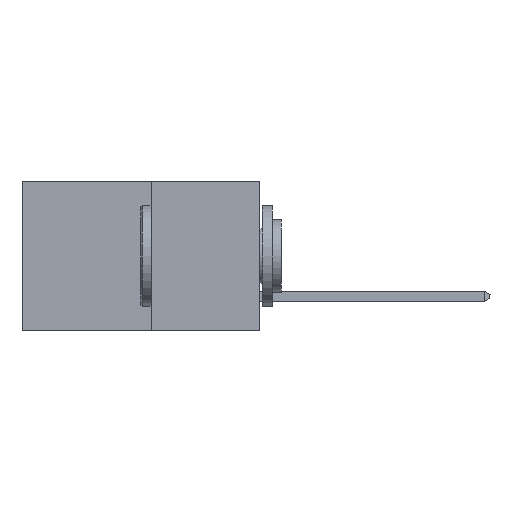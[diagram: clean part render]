
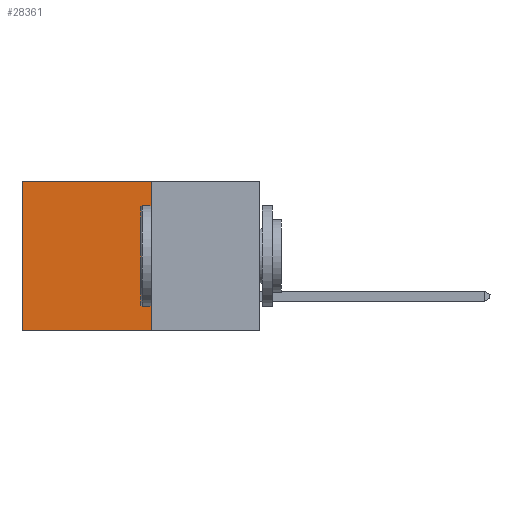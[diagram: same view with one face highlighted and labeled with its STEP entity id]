
A CAD part, left-side view. The second image highlights one B-rep face of the part: STEP entity #28361.
In plain terms, the highlighted planar face has unit normal (-1, 0, 0).
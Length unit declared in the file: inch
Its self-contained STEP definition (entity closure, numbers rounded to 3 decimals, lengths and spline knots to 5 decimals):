
#1286 = VERTEX_POINT ( 'NONE', #1595 ) ;
#1595 = CARTESIAN_POINT ( 'NONE',  ( 0.277, 0.27, 0. ) ) ;
#2074 = VECTOR ( 'NONE', #28582, 39.37008 ) ;
#3362 = LINE ( 'NONE', #7037, #16922 ) ;
#3975 = ORIENTED_EDGE ( 'NONE', *, *, #24869, .F. ) ;
#4629 = VERTEX_POINT ( 'NONE', #21192 ) ;
#6731 = ORIENTED_EDGE ( 'NONE', *, *, #15879, .T. ) ;
#6848 = DIRECTION ( 'NONE',  ( 0., 1., 0. ) ) ;
#7037 = CARTESIAN_POINT ( 'NONE',  ( 0.277, 0.27, 0. ) ) ;
#8183 = LINE ( 'NONE', #24771, #19464 ) ;
#8834 = LINE ( 'NONE', #11026, #2074 ) ;
#9857 = DIRECTION ( 'NONE',  ( 0., 0., -1. ) ) ;
#10007 = DIRECTION ( 'NONE',  ( 1., 0., 0. ) ) ;
#11014 = FACE_OUTER_BOUND ( 'NONE', #21969, .T. ) ;
#11026 = CARTESIAN_POINT ( 'NONE',  ( 0.277, 0.27, -0.37 ) ) ;
#12382 = AXIS2_PLACEMENT_3D ( 'NONE', #22544, #10007, #27489 ) ;
#12635 = EDGE_CURVE ( 'NONE', #30207, #19604, #8183, .T. ) ;
#13373 = ORIENTED_EDGE ( 'NONE', *, *, #16957, .F. ) ;
#15879 = EDGE_CURVE ( 'NONE', #1286, #30207, #3362, .T. ) ;
#16922 = VECTOR ( 'NONE', #17226, 39.37008 ) ;
#16957 = EDGE_CURVE ( 'NONE', #1286, #4629, #8834, .T. ) ;
#17226 = DIRECTION ( 'NONE',  ( 0., 1., 0. ) ) ;
#19464 = VECTOR ( 'NONE', #9857, 39.37008 ) ;
#19604 = VERTEX_POINT ( 'NONE', #22124 ) ;
#20611 = ORIENTED_EDGE ( 'NONE', *, *, #12635, .T. ) ;
#21192 = CARTESIAN_POINT ( 'NONE',  ( 0.277, 0.27, -0.37 ) ) ;
#21899 = VECTOR ( 'NONE', #6848, 39.37008 ) ;
#21969 = EDGE_LOOP ( 'NONE', ( #20611, #3975, #13373, #6731 ) ) ;
#22124 = CARTESIAN_POINT ( 'NONE',  ( 0.277, 0.59, -0.37 ) ) ;
#22544 = CARTESIAN_POINT ( 'NONE',  ( 0.277, 0.27, -0.37 ) ) ;
#22684 = CARTESIAN_POINT ( 'NONE',  ( 0.277, 0.59, 0. ) ) ;
#24371 = CARTESIAN_POINT ( 'NONE',  ( 0.277, 0.27, -0.37 ) ) ;
#24771 = CARTESIAN_POINT ( 'NONE',  ( 0.277, 0.59, -0.37 ) ) ;
#24869 = EDGE_CURVE ( 'NONE', #4629, #19604, #28430, .T. ) ;
#25036 = PLANE ( 'NONE',  #12382 ) ;
#27489 = DIRECTION ( 'NONE',  ( 0., 0., -1. ) ) ;
#28361 = ADVANCED_FACE ( 'NONE', ( #11014 ), #25036, .F. ) ;
#28430 = LINE ( 'NONE', #24371, #21899 ) ;
#28582 = DIRECTION ( 'NONE',  ( 0., 0., -1. ) ) ;
#30207 = VERTEX_POINT ( 'NONE', #22684 ) ;
